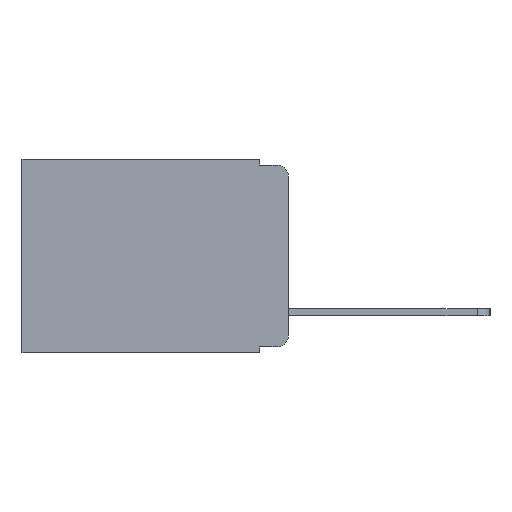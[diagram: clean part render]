
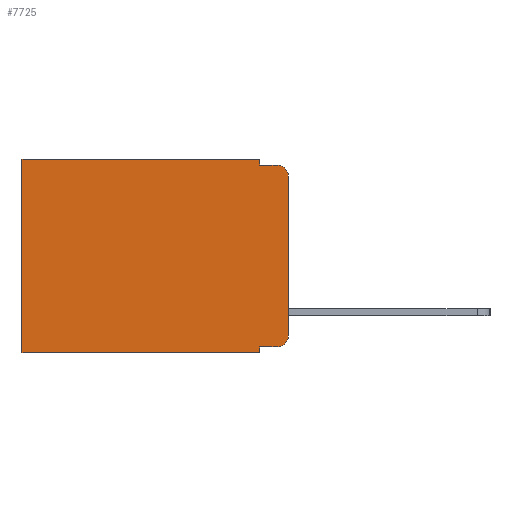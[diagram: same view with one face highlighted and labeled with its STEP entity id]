
A CAD part, left-side view. The second image highlights one B-rep face of the part: STEP entity #7725.
In plain terms, the highlighted planar face has unit normal (-1, 0, 0).
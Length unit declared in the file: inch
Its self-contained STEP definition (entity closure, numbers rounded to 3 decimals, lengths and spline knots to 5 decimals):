
#72 = CARTESIAN_POINT ( 'NONE',  ( 0.298, 0.051, 0. ) ) ;
#408 = EDGE_CURVE ( 'NONE', #5385, #8174, #2307, .T. ) ;
#490 = DIRECTION ( 'NONE',  ( 0., -1., 0. ) ) ;
#697 = CARTESIAN_POINT ( 'NONE',  ( 0.298, 0.051, 0. ) ) ;
#700 = CARTESIAN_POINT ( 'NONE',  ( 0.298, 0., 0. ) ) ;
#777 = CARTESIAN_POINT ( 'NONE',  ( 0.298, 0.02, -0.03 ) ) ;
#779 = LINE ( 'NONE', #697, #7226 ) ;
#836 = EDGE_CURVE ( 'NONE', #5635, #8083, #9654, .T. ) ;
#1043 = EDGE_CURVE ( 'NONE', #8083, #5638, #2854, .T. ) ;
#1135 = CARTESIAN_POINT ( 'NONE',  ( 0.298, 0.02, -0.313 ) ) ;
#1246 = LINE ( 'NONE', #700, #9752 ) ;
#1507 = VERTEX_POINT ( 'NONE', #5457 ) ;
#1541 = EDGE_CURVE ( 'NONE', #5635, #9259, #7744, .T. ) ;
#1738 = DIRECTION ( 'NONE',  ( 0., 0., -1. ) ) ;
#1757 = EDGE_CURVE ( 'NONE', #8915, #2501, #1246, .T. ) ;
#2079 = DIRECTION ( 'NONE',  ( 0., 0., -1. ) ) ;
#2307 = LINE ( 'NONE', #4408, #10927 ) ;
#2332 = DIRECTION ( 'NONE',  ( 0., -1., 0. ) ) ;
#2488 = ORIENTED_EDGE ( 'NONE', *, *, #836, .F. ) ;
#2501 = VERTEX_POINT ( 'NONE', #3879 ) ;
#2854 = LINE ( 'NONE', #10137, #9037 ) ;
#3201 = FACE_OUTER_BOUND ( 'NONE', #6795, .T. ) ;
#3852 = ORIENTED_EDGE ( 'NONE', *, *, #1043, .F. ) ;
#3879 = CARTESIAN_POINT ( 'NONE',  ( 0.298, 0., -0.313 ) ) ;
#3923 = DIRECTION ( 'NONE',  ( 0., 0., -1. ) ) ;
#3943 = CARTESIAN_POINT ( 'NONE',  ( 0.298, 0., 0. ) ) ;
#4251 = ORIENTED_EDGE ( 'NONE', *, *, #1757, .F. ) ;
#4408 = CARTESIAN_POINT ( 'NONE',  ( 0.298, 0., -0.343 ) ) ;
#4773 = CARTESIAN_POINT ( 'NONE',  ( 0.298, 0.473, 0. ) ) ;
#4842 = ORIENTED_EDGE ( 'NONE', *, *, #9989, .T. ) ;
#4862 = DIRECTION ( 'NONE',  ( 0., 0., -1. ) ) ;
#5097 = LINE ( 'NONE', #8931, #7308 ) ;
#5098 = ORIENTED_EDGE ( 'NONE', *, *, #408, .F. ) ;
#5385 = VERTEX_POINT ( 'NONE', #10811 ) ;
#5457 = CARTESIAN_POINT ( 'NONE',  ( 0.298, 0.051, -0.333 ) ) ;
#5490 = VERTEX_POINT ( 'NONE', #6139 ) ;
#5568 = VECTOR ( 'NONE', #10013, 39.37008 ) ;
#5623 = DIRECTION ( 'NONE',  ( 0., 1., 0. ) ) ;
#5635 = VERTEX_POINT ( 'NONE', #72 ) ;
#5638 = VERTEX_POINT ( 'NONE', #6330 ) ;
#5846 = DIRECTION ( 'NONE',  ( 0., 0., -1. ) ) ;
#6138 = CIRCLE ( 'NONE', #9634, 0.02 ) ;
#6139 = CARTESIAN_POINT ( 'NONE',  ( 0.298, 0.02, -0.333 ) ) ;
#6330 = CARTESIAN_POINT ( 'NONE',  ( 0.298, 0.02, -0.01 ) ) ;
#6452 = LINE ( 'NONE', #7463, #8858 ) ;
#6749 = EDGE_CURVE ( 'NONE', #1507, #5385, #779, .T. ) ;
#6795 = EDGE_LOOP ( 'NONE', ( #4251, #10829, #3852, #2488, #7054, #4842, #5098, #9203, #9452, #7310 ) ) ;
#6938 = DIRECTION ( 'NONE',  ( -1., 0., 0. ) ) ;
#7054 = ORIENTED_EDGE ( 'NONE', *, *, #1541, .T. ) ;
#7226 = VECTOR ( 'NONE', #7679, 39.37008 ) ;
#7236 = DIRECTION ( 'NONE',  ( -1., 0., 0. ) ) ;
#7308 = VECTOR ( 'NONE', #3923, 39.37008 ) ;
#7310 = ORIENTED_EDGE ( 'NONE', *, *, #8393, .T. ) ;
#7320 = PLANE ( 'NONE',  #10757 ) ;
#7463 = CARTESIAN_POINT ( 'NONE',  ( 0.298, 0.051, -0.333 ) ) ;
#7515 = VECTOR ( 'NONE', #5846, 39.37008 ) ;
#7679 = DIRECTION ( 'NONE',  ( 0., 0., -1. ) ) ;
#7725 = ADVANCED_FACE ( 'NONE', ( #3201 ), #7320, .F. ) ;
#7744 = LINE ( 'NONE', #10898, #5568 ) ;
#7827 = EDGE_CURVE ( 'NONE', #1507, #5490, #6452, .T. ) ;
#7884 = CARTESIAN_POINT ( 'NONE',  ( 0.298, 0.051, 0. ) ) ;
#8083 = VERTEX_POINT ( 'NONE', #10939 ) ;
#8174 = VERTEX_POINT ( 'NONE', #9432 ) ;
#8393 = EDGE_CURVE ( 'NONE', #5490, #2501, #10978, .T. ) ;
#8858 = VECTOR ( 'NONE', #2332, 39.37008 ) ;
#8915 = VERTEX_POINT ( 'NONE', #10877 ) ;
#8931 = CARTESIAN_POINT ( 'NONE',  ( 0.298, 0.473, 0. ) ) ;
#9037 = VECTOR ( 'NONE', #490, 39.37008 ) ;
#9203 = ORIENTED_EDGE ( 'NONE', *, *, #6749, .F. ) ;
#9259 = VERTEX_POINT ( 'NONE', #4773 ) ;
#9432 = CARTESIAN_POINT ( 'NONE',  ( 0.298, 0.473, -0.343 ) ) ;
#9452 = ORIENTED_EDGE ( 'NONE', *, *, #7827, .T. ) ;
#9634 = AXIS2_PLACEMENT_3D ( 'NONE', #777, #6938, #1738 ) ;
#9654 = LINE ( 'NONE', #7884, #7515 ) ;
#9746 = DIRECTION ( 'NONE',  ( 1., 0., 0. ) ) ;
#9752 = VECTOR ( 'NONE', #10020, 39.37008 ) ;
#9989 = EDGE_CURVE ( 'NONE', #9259, #8174, #5097, .T. ) ;
#10013 = DIRECTION ( 'NONE',  ( 0., 1., 0. ) ) ;
#10020 = DIRECTION ( 'NONE',  ( 0., 0., -1. ) ) ;
#10137 = CARTESIAN_POINT ( 'NONE',  ( 0.298, 0.051, -0.01 ) ) ;
#10362 = EDGE_CURVE ( 'NONE', #8915, #5638, #6138, .T. ) ;
#10757 = AXIS2_PLACEMENT_3D ( 'NONE', #3943, #9746, #4862 ) ;
#10811 = CARTESIAN_POINT ( 'NONE',  ( 0.298, 0.051, -0.343 ) ) ;
#10829 = ORIENTED_EDGE ( 'NONE', *, *, #10362, .T. ) ;
#10877 = CARTESIAN_POINT ( 'NONE',  ( 0.298, 0., -0.03 ) ) ;
#10898 = CARTESIAN_POINT ( 'NONE',  ( 0.298, 0., 0. ) ) ;
#10927 = VECTOR ( 'NONE', #5623, 39.37008 ) ;
#10939 = CARTESIAN_POINT ( 'NONE',  ( 0.298, 0.051, -0.01 ) ) ;
#10978 = CIRCLE ( 'NONE', #11041, 0.02 ) ;
#11041 = AXIS2_PLACEMENT_3D ( 'NONE', #1135, #7236, #2079 ) ;
